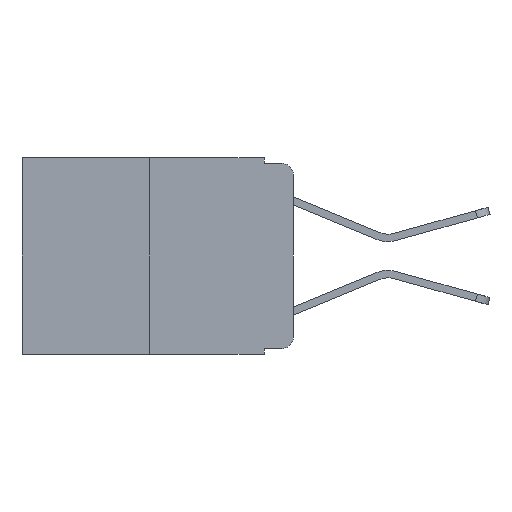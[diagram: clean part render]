
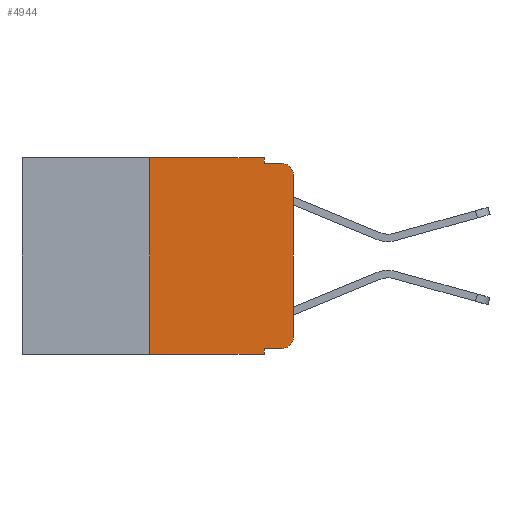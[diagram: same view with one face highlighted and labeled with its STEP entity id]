
A CAD part, left-side view. The second image highlights one B-rep face of the part: STEP entity #4944.
In plain terms, the highlighted planar face has unit normal (-1, 0, 0).
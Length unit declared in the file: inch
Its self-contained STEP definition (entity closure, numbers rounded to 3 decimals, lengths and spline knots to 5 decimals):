
#136 = CARTESIAN_POINT ( 'NONE',  ( 0., 0.473, -0.343 ) ) ;
#160 = LINE ( 'NONE', #6002, #4517 ) ;
#485 = VERTEX_POINT ( 'NONE', #5468 ) ;
#650 = ORIENTED_EDGE ( 'NONE', *, *, #3124, .F. ) ;
#651 = DIRECTION ( 'NONE',  ( 0., -1., 0. ) ) ;
#784 = DIRECTION ( 'NONE',  ( 0., 0., -1. ) ) ;
#789 = ORIENTED_EDGE ( 'NONE', *, *, #4208, .F. ) ;
#805 = DIRECTION ( 'NONE',  ( 0., 0., 1. ) ) ;
#832 = DIRECTION ( 'NONE',  ( 0., -1., 0. ) ) ;
#893 = VERTEX_POINT ( 'NONE', #4538 ) ;
#906 = ORIENTED_EDGE ( 'NONE', *, *, #1370, .T. ) ;
#917 = ORIENTED_EDGE ( 'NONE', *, *, #3688, .F. ) ;
#1264 = ORIENTED_EDGE ( 'NONE', *, *, #1974, .F. ) ;
#1294 = ORIENTED_EDGE ( 'NONE', *, *, #4665, .T. ) ;
#1370 = EDGE_CURVE ( 'NONE', #3732, #5308, #3869, .T. ) ;
#1407 = LINE ( 'NONE', #8428, #8604 ) ;
#1599 = PLANE ( 'NONE',  #5635 ) ;
#1796 = DIRECTION ( 'NONE',  ( -1., 0., 0. ) ) ;
#1859 = DIRECTION ( 'NONE',  ( 0., -1., 0. ) ) ;
#1974 = EDGE_CURVE ( 'NONE', #485, #7963, #8220, .T. ) ;
#1999 = ORIENTED_EDGE ( 'NONE', *, *, #2123, .T. ) ;
#2034 = EDGE_CURVE ( 'NONE', #8597, #3732, #160, .T. ) ;
#2123 = EDGE_CURVE ( 'NONE', #6724, #3479, #4092, .T. ) ;
#2133 = CARTESIAN_POINT ( 'NONE',  ( 0., 0.051, -0.343 ) ) ;
#2173 = VECTOR ( 'NONE', #2796, 39.37008 ) ;
#2590 = EDGE_CURVE ( 'NONE', #8597, #3479, #7844, .T. ) ;
#2718 = ORIENTED_EDGE ( 'NONE', *, *, #5134, .T. ) ;
#2774 = LINE ( 'NONE', #3772, #4596 ) ;
#2796 = DIRECTION ( 'NONE',  ( 0., 0., -1. ) ) ;
#2819 = AXIS2_PLACEMENT_3D ( 'NONE', #5046, #1796, #5180 ) ;
#3008 = CARTESIAN_POINT ( 'NONE',  ( 0., 0.02, -0.333 ) ) ;
#3027 = CARTESIAN_POINT ( 'NONE',  ( 0., 0.051, 0. ) ) ;
#3124 = EDGE_CURVE ( 'NONE', #6724, #485, #1407, .T. ) ;
#3388 = FACE_OUTER_BOUND ( 'NONE', #4429, .T. ) ;
#3479 = VERTEX_POINT ( 'NONE', #2133 ) ;
#3498 = VERTEX_POINT ( 'NONE', #8315 ) ;
#3688 = EDGE_CURVE ( 'NONE', #7963, #7162, #6013, .T. ) ;
#3732 = VERTEX_POINT ( 'NONE', #3008 ) ;
#3772 = CARTESIAN_POINT ( 'NONE',  ( 0., 0.051, -0.01 ) ) ;
#3869 = CIRCLE ( 'NONE', #6279, 0.02 ) ;
#4092 = LINE ( 'NONE', #136, #7454 ) ;
#4130 = DIRECTION ( 'NONE',  ( 0., 0., 1. ) ) ;
#4208 = EDGE_CURVE ( 'NONE', #7162, #3498, #2774, .T. ) ;
#4429 = EDGE_LOOP ( 'NONE', ( #2718, #1294, #789, #917, #1264, #650, #1999, #6823, #4622, #906 ) ) ;
#4457 = CARTESIAN_POINT ( 'NONE',  ( 0., 0., 0. ) ) ;
#4517 = VECTOR ( 'NONE', #8024, 39.37008 ) ;
#4538 = CARTESIAN_POINT ( 'NONE',  ( 0., 0., -0.03 ) ) ;
#4596 = VECTOR ( 'NONE', #1859, 39.37008 ) ;
#4622 = ORIENTED_EDGE ( 'NONE', *, *, #2034, .T. ) ;
#4665 = EDGE_CURVE ( 'NONE', #893, #3498, #7006, .T. ) ;
#4929 = CARTESIAN_POINT ( 'NONE',  ( 0., 0.25, -0.343 ) ) ;
#4944 = ADVANCED_FACE ( 'NONE', ( #3388 ), #1599, .F. ) ;
#4951 = CARTESIAN_POINT ( 'NONE',  ( 0., 0.051, 0. ) ) ;
#5046 = CARTESIAN_POINT ( 'NONE',  ( 0., 0.02, -0.03 ) ) ;
#5134 = EDGE_CURVE ( 'NONE', #5308, #893, #5878, .T. ) ;
#5180 = DIRECTION ( 'NONE',  ( 0., 0., -1. ) ) ;
#5293 = CARTESIAN_POINT ( 'NONE',  ( 0., 0.051, -0.01 ) ) ;
#5308 = VERTEX_POINT ( 'NONE', #8606 ) ;
#5468 = CARTESIAN_POINT ( 'NONE',  ( 0., 0.25, 0. ) ) ;
#5635 = AXIS2_PLACEMENT_3D ( 'NONE', #8026, #6022, #6155 ) ;
#5878 = LINE ( 'NONE', #4457, #7619 ) ;
#5899 = CARTESIAN_POINT ( 'NONE',  ( 0., 0.051, 0. ) ) ;
#6002 = CARTESIAN_POINT ( 'NONE',  ( 0., 0.051, -0.333 ) ) ;
#6013 = LINE ( 'NONE', #4951, #7540 ) ;
#6022 = DIRECTION ( 'NONE',  ( 1., 0., 0. ) ) ;
#6155 = DIRECTION ( 'NONE',  ( 0., 0., -1. ) ) ;
#6274 = DIRECTION ( 'NONE',  ( 0., 0., -1. ) ) ;
#6279 = AXIS2_PLACEMENT_3D ( 'NONE', #6719, #6635, #784 ) ;
#6531 = VECTOR ( 'NONE', #651, 39.37008 ) ;
#6635 = DIRECTION ( 'NONE',  ( -1., 0., 0. ) ) ;
#6719 = CARTESIAN_POINT ( 'NONE',  ( 0., 0.02, -0.313 ) ) ;
#6724 = VERTEX_POINT ( 'NONE', #4929 ) ;
#6823 = ORIENTED_EDGE ( 'NONE', *, *, #2590, .F. ) ;
#7006 = CIRCLE ( 'NONE', #2819, 0.02 ) ;
#7158 = CARTESIAN_POINT ( 'NONE',  ( 0., 0.473, 0. ) ) ;
#7162 = VERTEX_POINT ( 'NONE', #5293 ) ;
#7454 = VECTOR ( 'NONE', #832, 39.37008 ) ;
#7540 = VECTOR ( 'NONE', #6274, 39.37008 ) ;
#7619 = VECTOR ( 'NONE', #4130, 39.37008 ) ;
#7844 = LINE ( 'NONE', #5899, #2173 ) ;
#7963 = VERTEX_POINT ( 'NONE', #3027 ) ;
#8024 = DIRECTION ( 'NONE',  ( 0., -1., 0. ) ) ;
#8026 = CARTESIAN_POINT ( 'NONE',  ( 0., 0.473, 0. ) ) ;
#8220 = LINE ( 'NONE', #7158, #6531 ) ;
#8315 = CARTESIAN_POINT ( 'NONE',  ( 0., 0.02, -0.01 ) ) ;
#8428 = CARTESIAN_POINT ( 'NONE',  ( 0., 0.25, 0. ) ) ;
#8597 = VERTEX_POINT ( 'NONE', #8983 ) ;
#8604 = VECTOR ( 'NONE', #805, 39.37008 ) ;
#8606 = CARTESIAN_POINT ( 'NONE',  ( 0., 0., -0.313 ) ) ;
#8983 = CARTESIAN_POINT ( 'NONE',  ( 0., 0.051, -0.333 ) ) ;
